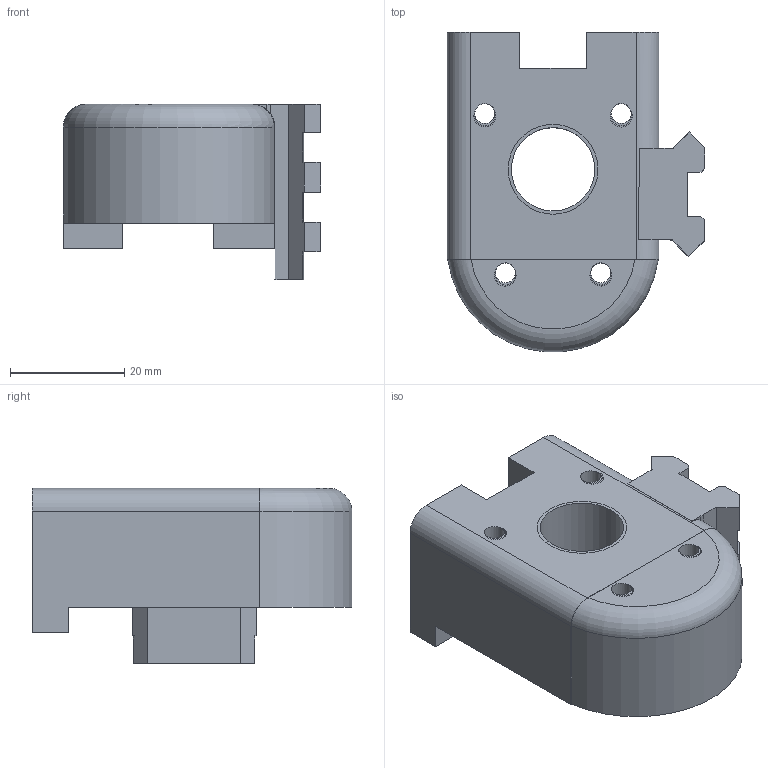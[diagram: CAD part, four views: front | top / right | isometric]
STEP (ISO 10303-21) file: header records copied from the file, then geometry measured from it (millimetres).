
FILE_DESCRIPTION(('FreeCAD Model'),'2;1');
FILE_NAME('ap9 barrel retainer 2020.step','2020-04-04T17:36:33',('Author'),(''), 'Open CASCADE STEP processor 6.8','FreeCAD','Unknown');
FILE_SCHEMA(('AUTOMOTIVE_DESIGN_CC2 { 1 2 10303 214 -1 1 5 4 }'));
Length unit declared in the file: millimetre
Products named in the file (1): Pocket025
Bounding box: 45.13 x 55.95 x 30.73 mm (x, y, z)
Volume: 37508 mm3; surface area: 10640.6 mm2
Topology: 1 solids, 2 shells, 131 faces, 393 edges, 269 vertices
Faces by surface type: plane 114, cylinder 16, torus 1
Full cylindrical faces by diameter (mm): 3.5 x4, 14.6 x1
Entity records: 10450 total; most frequent: CARTESIAN_POINT 2950, DIRECTION 1333, LINE 826, VECTOR 826, ORIENTED_EDGE 786, PCURVE 786, DEFINITIONAL_REPRESENTATION 786, EDGE_CURVE 393
